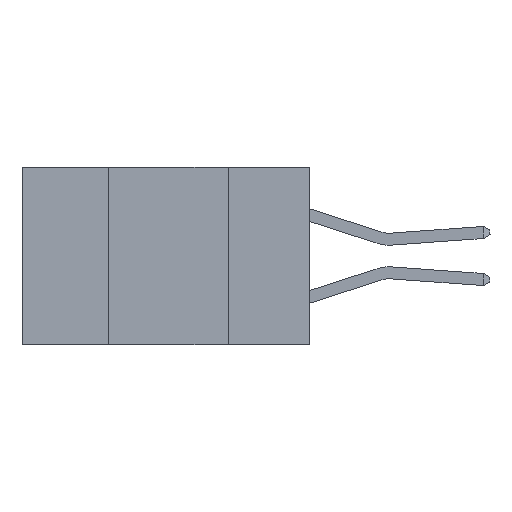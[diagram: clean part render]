
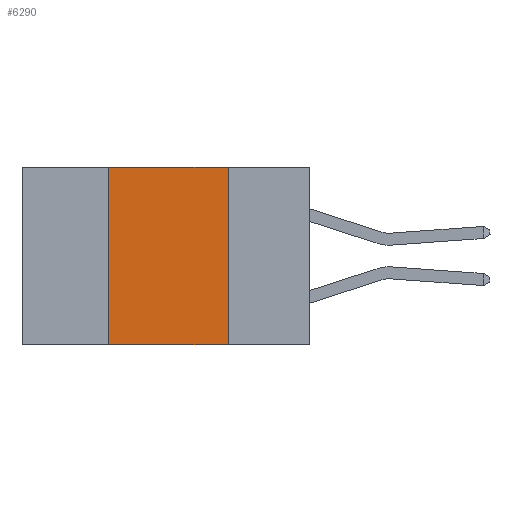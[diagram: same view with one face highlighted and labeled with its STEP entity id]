
A CAD part, left-side view. The second image highlights one B-rep face of the part: STEP entity #6290.
In plain terms, the highlighted planar face has unit normal (-1, 0, 0).
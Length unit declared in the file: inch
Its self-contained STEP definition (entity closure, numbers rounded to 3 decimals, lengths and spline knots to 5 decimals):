
#592 = CARTESIAN_POINT ( 'NONE',  ( 0., 0.17, -0.37 ) ) ;
#808 = VERTEX_POINT ( 'NONE', #11840 ) ;
#928 = LINE ( 'NONE', #20954, #9872 ) ;
#1252 = DIRECTION ( 'NONE',  ( 0., -1., 0. ) ) ;
#2108 = CARTESIAN_POINT ( 'NONE',  ( 0., 0.17, -0.37 ) ) ;
#2512 = VERTEX_POINT ( 'NONE', #6082 ) ;
#2672 = EDGE_CURVE ( 'NONE', #808, #6535, #5198, .T. ) ;
#3652 = CARTESIAN_POINT ( 'NONE',  ( 0., 0.17, 0. ) ) ;
#3985 = AXIS2_PLACEMENT_3D ( 'NONE', #4303, #15104, #11608 ) ;
#4229 = ORIENTED_EDGE ( 'NONE', *, *, #18049, .F. ) ;
#4303 = CARTESIAN_POINT ( 'NONE',  ( 0., 0.6, 0. ) ) ;
#4687 = LINE ( 'NONE', #14153, #7074 ) ;
#4750 = DIRECTION ( 'NONE',  ( 0., 0., 1. ) ) ;
#4888 = VECTOR ( 'NONE', #1252, 39.37008 ) ;
#4923 = DIRECTION ( 'NONE',  ( 0., -1., 0. ) ) ;
#5198 = LINE ( 'NONE', #17702, #4888 ) ;
#5982 = PLANE ( 'NONE',  #3985 ) ;
#6082 = CARTESIAN_POINT ( 'NONE',  ( 0., 0.42, 0. ) ) ;
#6290 = ADVANCED_FACE ( 'NONE', ( #15218 ), #5982, .F. ) ;
#6535 = VERTEX_POINT ( 'NONE', #2108 ) ;
#7074 = VECTOR ( 'NONE', #4923, 39.37008 ) ;
#7784 = EDGE_CURVE ( 'NONE', #2512, #8866, #4687, .T. ) ;
#8481 = EDGE_LOOP ( 'NONE', ( #12605, #22975, #4229, #9914 ) ) ;
#8866 = VERTEX_POINT ( 'NONE', #3652 ) ;
#9872 = VECTOR ( 'NONE', #4750, 39.37008 ) ;
#9914 = ORIENTED_EDGE ( 'NONE', *, *, #2672, .T. ) ;
#11608 = DIRECTION ( 'NONE',  ( 0., 0., -1. ) ) ;
#11840 = CARTESIAN_POINT ( 'NONE',  ( 0., 0.42, -0.37 ) ) ;
#12605 = ORIENTED_EDGE ( 'NONE', *, *, #16427, .F. ) ;
#14153 = CARTESIAN_POINT ( 'NONE',  ( 0., 0.6, 0. ) ) ;
#15000 = LINE ( 'NONE', #592, #20913 ) ;
#15104 = DIRECTION ( 'NONE',  ( 1., 0., 0. ) ) ;
#15218 = FACE_OUTER_BOUND ( 'NONE', #8481, .T. ) ;
#16427 = EDGE_CURVE ( 'NONE', #8866, #6535, #15000, .T. ) ;
#17702 = CARTESIAN_POINT ( 'NONE',  ( 0., 0.6, -0.37 ) ) ;
#18049 = EDGE_CURVE ( 'NONE', #808, #2512, #928, .T. ) ;
#18475 = DIRECTION ( 'NONE',  ( 0., 0., -1. ) ) ;
#20913 = VECTOR ( 'NONE', #18475, 39.37008 ) ;
#20954 = CARTESIAN_POINT ( 'NONE',  ( 0., 0.42, -0.37 ) ) ;
#22975 = ORIENTED_EDGE ( 'NONE', *, *, #7784, .F. ) ;
